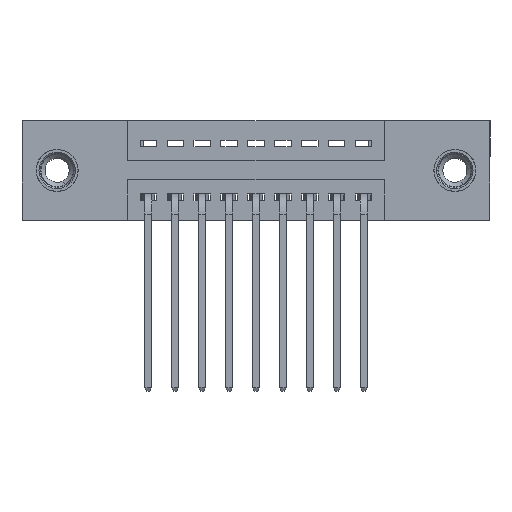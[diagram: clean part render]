
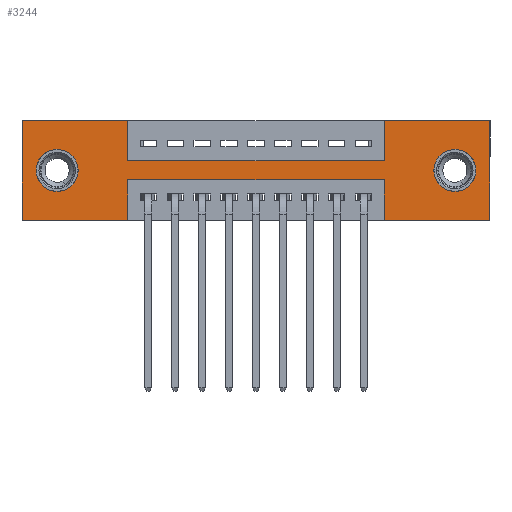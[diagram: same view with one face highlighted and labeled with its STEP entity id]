
A CAD part, front view. The second image highlights one B-rep face of the part: STEP entity #3244.
In plain terms, the highlighted planar face has unit normal (0, -1, 0).
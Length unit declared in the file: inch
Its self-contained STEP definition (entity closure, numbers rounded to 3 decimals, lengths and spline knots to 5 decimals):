
#13 = ORIENTED_EDGE ( 'NONE', *, *, #15311, .T. ) ;
#126 = DIRECTION ( 'NONE',  ( 0., 0., 1. ) ) ;
#470 = ORIENTED_EDGE ( 'NONE', *, *, #9183, .T. ) ;
#475 = VERTEX_POINT ( 'NONE', #809 ) ;
#561 = DIRECTION ( 'NONE',  ( 0., 1., 0. ) ) ;
#603 = CARTESIAN_POINT ( 'NONE',  ( 1.735, 0., 0. ) ) ;
#607 = VECTOR ( 'NONE', #3544, 39.37008 ) ;
#634 = DIRECTION ( 'NONE',  ( 1., 0., 0. ) ) ;
#748 = LINE ( 'NONE', #6832, #9469 ) ;
#809 = CARTESIAN_POINT ( 'NONE',  ( 1.3425, 0., -0.22 ) ) ;
#852 = DIRECTION ( 'NONE',  ( 1., 0., 0. ) ) ;
#900 = CARTESIAN_POINT ( 'NONE',  ( 0.3925, 0., -0.15 ) ) ;
#1021 = LINE ( 'NONE', #3330, #607 ) ;
#1169 = PLANE ( 'NONE',  #15642 ) ;
#1269 = VERTEX_POINT ( 'NONE', #4388 ) ;
#1323 = DIRECTION ( 'NONE',  ( 0., 0., 1. ) ) ;
#1399 = DIRECTION ( 'NONE',  ( 1., 0., 0. ) ) ;
#1473 = VECTOR ( 'NONE', #1476, 39.37008 ) ;
#1476 = DIRECTION ( 'NONE',  ( -1., 0., 0. ) ) ;
#1689 = CARTESIAN_POINT ( 'NONE',  ( 0., 0., 0. ) ) ;
#1809 = DIRECTION ( 'NONE',  ( 0., 0., -1. ) ) ;
#1827 = CIRCLE ( 'NONE', #7024, 0.078 ) ;
#1872 = EDGE_CURVE ( 'NONE', #475, #8983, #9432, .T. ) ;
#1948 = VECTOR ( 'NONE', #126, 39.37008 ) ;
#1971 = DIRECTION ( 'NONE',  ( 0., 1., 0. ) ) ;
#1984 = ORIENTED_EDGE ( 'NONE', *, *, #5284, .F. ) ;
#2063 = VERTEX_POINT ( 'NONE', #4811 ) ;
#2188 = CARTESIAN_POINT ( 'NONE',  ( 1.735, 0., -0.37 ) ) ;
#2365 = CARTESIAN_POINT ( 'NONE',  ( 1.605, 0., -0.107 ) ) ;
#2401 = DIRECTION ( 'NONE',  ( 0., 0., -1. ) ) ;
#2526 = EDGE_LOOP ( 'NONE', ( #5293, #15737, #3232, #7009, #10838, #7139, #11285, #9414, #4150, #3745, #1984, #12506 ) ) ;
#2564 = LINE ( 'NONE', #3757, #15328 ) ;
#2954 = EDGE_CURVE ( 'NONE', #9020, #9436, #6504, .T. ) ;
#3002 = EDGE_CURVE ( 'NONE', #9436, #11527, #9780, .T. ) ;
#3119 = VERTEX_POINT ( 'NONE', #2188 ) ;
#3232 = ORIENTED_EDGE ( 'NONE', *, *, #9099, .F. ) ;
#3244 = ADVANCED_FACE ( 'NONE', ( #4140, #7663, #12317 ), #1169, .T. ) ;
#3255 = LINE ( 'NONE', #13744, #16060 ) ;
#3330 = CARTESIAN_POINT ( 'NONE',  ( 1.3425, 0., 0. ) ) ;
#3544 = DIRECTION ( 'NONE',  ( 0., 0., 1. ) ) ;
#3550 = CARTESIAN_POINT ( 'NONE',  ( 0., 0., -0.37 ) ) ;
#3551 = CARTESIAN_POINT ( 'NONE',  ( 0.13, 0., -0.185 ) ) ;
#3745 = ORIENTED_EDGE ( 'NONE', *, *, #7571, .F. ) ;
#3757 = CARTESIAN_POINT ( 'NONE',  ( 0., 0., -0.37 ) ) ;
#4083 = CARTESIAN_POINT ( 'NONE',  ( 0.13, 0., -0.185 ) ) ;
#4140 = FACE_BOUND ( 'NONE', #16039, .T. ) ;
#4150 = ORIENTED_EDGE ( 'NONE', *, *, #2954, .F. ) ;
#4243 = CARTESIAN_POINT ( 'NONE',  ( 0.3925, 0., -0.22 ) ) ;
#4388 = CARTESIAN_POINT ( 'NONE',  ( 1.3425, 0., -0.37 ) ) ;
#4543 = CARTESIAN_POINT ( 'NONE',  ( 0.3925, 0., -0.22 ) ) ;
#4609 = EDGE_CURVE ( 'NONE', #11527, #6694, #1021, .T. ) ;
#4734 = EDGE_CURVE ( 'NONE', #10628, #15154, #2564, .T. ) ;
#4811 = CARTESIAN_POINT ( 'NONE',  ( 1.605, 0., -0.263 ) ) ;
#4863 = DIRECTION ( 'NONE',  ( -1., 0., 0. ) ) ;
#4960 = CIRCLE ( 'NONE', #5891, 0.078 ) ;
#4995 = CARTESIAN_POINT ( 'NONE',  ( 0.3925, 0., -0.15 ) ) ;
#5056 = ORIENTED_EDGE ( 'NONE', *, *, #15333, .T. ) ;
#5084 = CARTESIAN_POINT ( 'NONE',  ( 1.3425, 0., -0.37 ) ) ;
#5284 = EDGE_CURVE ( 'NONE', #15154, #10702, #13205, .T. ) ;
#5293 = ORIENTED_EDGE ( 'NONE', *, *, #6511, .F. ) ;
#5345 = DIRECTION ( 'NONE',  ( 0., 0., 1. ) ) ;
#5405 = CARTESIAN_POINT ( 'NONE',  ( 0.3925, 0., -0.37 ) ) ;
#5660 = AXIS2_PLACEMENT_3D ( 'NONE', #3551, #6116, #1323 ) ;
#5748 = VECTOR ( 'NONE', #15504, 39.37008 ) ;
#5860 = CARTESIAN_POINT ( 'NONE',  ( 0.3925, 0., 0. ) ) ;
#5891 = AXIS2_PLACEMENT_3D ( 'NONE', #4083, #12771, #5345 ) ;
#6023 = LINE ( 'NONE', #15623, #11619 ) ;
#6116 = DIRECTION ( 'NONE',  ( 0., 1., 0. ) ) ;
#6504 = LINE ( 'NONE', #5860, #5748 ) ;
#6511 = EDGE_CURVE ( 'NONE', #8983, #10628, #6023, .T. ) ;
#6604 = VERTEX_POINT ( 'NONE', #15953 ) ;
#6694 = VERTEX_POINT ( 'NONE', #8918 ) ;
#6832 = CARTESIAN_POINT ( 'NONE',  ( 0., 0., 0. ) ) ;
#7009 = ORIENTED_EDGE ( 'NONE', *, *, #8888, .F. ) ;
#7024 = AXIS2_PLACEMENT_3D ( 'NONE', #8000, #561, #1809 ) ;
#7139 = ORIENTED_EDGE ( 'NONE', *, *, #7394, .F. ) ;
#7183 = LINE ( 'NONE', #603, #13937 ) ;
#7252 = EDGE_LOOP ( 'NONE', ( #470, #12439 ) ) ;
#7394 = EDGE_CURVE ( 'NONE', #6694, #6604, #3255, .T. ) ;
#7571 = EDGE_CURVE ( 'NONE', #10702, #9020, #748, .T. ) ;
#7663 = FACE_BOUND ( 'NONE', #7252, .T. ) ;
#8000 = CARTESIAN_POINT ( 'NONE',  ( 1.605, 0., -0.185 ) ) ;
#8067 = LINE ( 'NONE', #11295, #1473 ) ;
#8613 = VECTOR ( 'NONE', #852, 39.37008 ) ;
#8888 = EDGE_CURVE ( 'NONE', #3119, #1269, #8067, .T. ) ;
#8918 = CARTESIAN_POINT ( 'NONE',  ( 1.3425, 0., 0. ) ) ;
#8983 = VERTEX_POINT ( 'NONE', #4243 ) ;
#9020 = VERTEX_POINT ( 'NONE', #11569 ) ;
#9042 = CARTESIAN_POINT ( 'NONE',  ( 0., 0., -0.37 ) ) ;
#9099 = EDGE_CURVE ( 'NONE', #1269, #475, #11733, .T. ) ;
#9183 = EDGE_CURVE ( 'NONE', #15345, #14187, #4960, .T. ) ;
#9197 = CARTESIAN_POINT ( 'NONE',  ( 1.3425, 0., -0.15 ) ) ;
#9414 = ORIENTED_EDGE ( 'NONE', *, *, #3002, .F. ) ;
#9432 = LINE ( 'NONE', #4543, #15029 ) ;
#9436 = VERTEX_POINT ( 'NONE', #4995 ) ;
#9469 = VECTOR ( 'NONE', #634, 39.37008 ) ;
#9780 = LINE ( 'NONE', #900, #8613 ) ;
#9789 = VECTOR ( 'NONE', #13730, 39.37008 ) ;
#9827 = DIRECTION ( 'NONE',  ( 0., -1., 0. ) ) ;
#10067 = EDGE_CURVE ( 'NONE', #14187, #15345, #11897, .T. ) ;
#10106 = AXIS2_PLACEMENT_3D ( 'NONE', #10463, #1971, #10515 ) ;
#10463 = CARTESIAN_POINT ( 'NONE',  ( 1.605, 0., -0.185 ) ) ;
#10515 = DIRECTION ( 'NONE',  ( 0., 0., -1. ) ) ;
#10628 = VERTEX_POINT ( 'NONE', #5405 ) ;
#10702 = VERTEX_POINT ( 'NONE', #1689 ) ;
#10809 = DIRECTION ( 'NONE',  ( 0., 0., -1. ) ) ;
#10838 = ORIENTED_EDGE ( 'NONE', *, *, #12584, .F. ) ;
#11194 = CARTESIAN_POINT ( 'NONE',  ( 0., 0., 0. ) ) ;
#11285 = ORIENTED_EDGE ( 'NONE', *, *, #4609, .F. ) ;
#11295 = CARTESIAN_POINT ( 'NONE',  ( 0., 0., -0.37 ) ) ;
#11527 = VERTEX_POINT ( 'NONE', #9197 ) ;
#11569 = CARTESIAN_POINT ( 'NONE',  ( 0.3925, 0., 0. ) ) ;
#11619 = VECTOR ( 'NONE', #10809, 39.37008 ) ;
#11733 = LINE ( 'NONE', #5084, #9789 ) ;
#11897 = CIRCLE ( 'NONE', #5660, 0.078 ) ;
#12125 = CARTESIAN_POINT ( 'NONE',  ( 0.13, 0., -0.107 ) ) ;
#12314 = CIRCLE ( 'NONE', #10106, 0.078 ) ;
#12317 = FACE_OUTER_BOUND ( 'NONE', #2526, .T. ) ;
#12439 = ORIENTED_EDGE ( 'NONE', *, *, #10067, .T. ) ;
#12506 = ORIENTED_EDGE ( 'NONE', *, *, #4734, .F. ) ;
#12584 = EDGE_CURVE ( 'NONE', #6604, #3119, #7183, .T. ) ;
#12771 = DIRECTION ( 'NONE',  ( 0., 1., 0. ) ) ;
#13021 = DIRECTION ( 'NONE',  ( 0., 0., -1. ) ) ;
#13100 = DIRECTION ( 'NONE',  ( -1., 0., 0. ) ) ;
#13205 = LINE ( 'NONE', #11194, #1948 ) ;
#13210 = CARTESIAN_POINT ( 'NONE',  ( 0.13, 0., -0.263 ) ) ;
#13730 = DIRECTION ( 'NONE',  ( 0., 0., 1. ) ) ;
#13744 = CARTESIAN_POINT ( 'NONE',  ( 0., 0., 0. ) ) ;
#13937 = VECTOR ( 'NONE', #13021, 39.37008 ) ;
#14187 = VERTEX_POINT ( 'NONE', #13210 ) ;
#15029 = VECTOR ( 'NONE', #13100, 39.37008 ) ;
#15154 = VERTEX_POINT ( 'NONE', #9042 ) ;
#15311 = EDGE_CURVE ( 'NONE', #2063, #15923, #12314, .T. ) ;
#15328 = VECTOR ( 'NONE', #4863, 39.37008 ) ;
#15333 = EDGE_CURVE ( 'NONE', #15923, #2063, #1827, .T. ) ;
#15345 = VERTEX_POINT ( 'NONE', #12125 ) ;
#15504 = DIRECTION ( 'NONE',  ( 0., 0., -1. ) ) ;
#15623 = CARTESIAN_POINT ( 'NONE',  ( 0.3925, 0., -0.37 ) ) ;
#15642 = AXIS2_PLACEMENT_3D ( 'NONE', #3550, #9827, #2401 ) ;
#15737 = ORIENTED_EDGE ( 'NONE', *, *, #1872, .F. ) ;
#15923 = VERTEX_POINT ( 'NONE', #2365 ) ;
#15953 = CARTESIAN_POINT ( 'NONE',  ( 1.735, 0., 0. ) ) ;
#16039 = EDGE_LOOP ( 'NONE', ( #5056, #13 ) ) ;
#16060 = VECTOR ( 'NONE', #1399, 39.37008 ) ;
